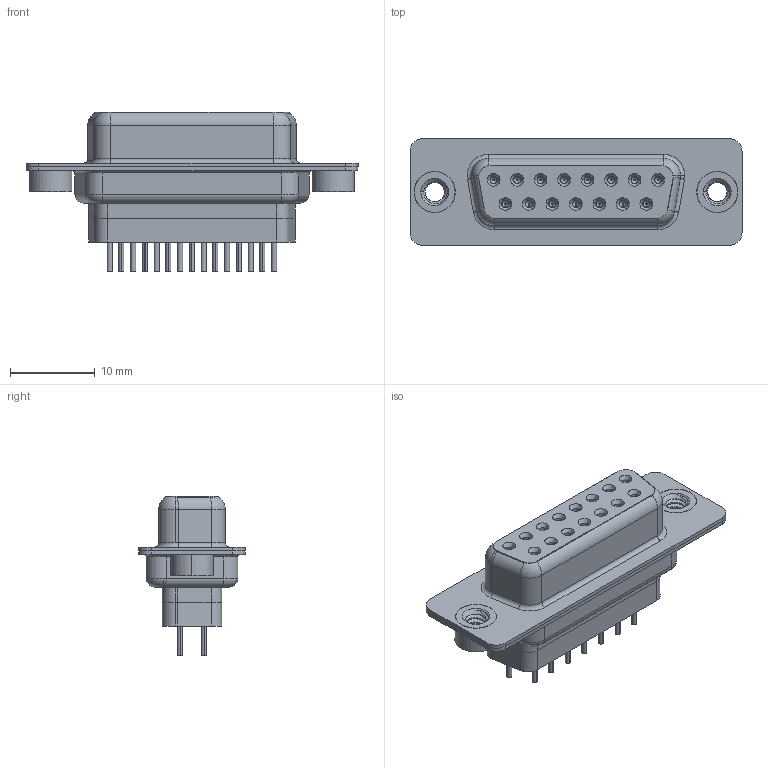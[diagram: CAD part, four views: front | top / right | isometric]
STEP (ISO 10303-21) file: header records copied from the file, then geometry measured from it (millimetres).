
FILE_DESCRIPTION (( 'STEP AP203' ), '1' );
FILE_NAME ('628-015-228-262.STEP', '2020-07-20T23:10:51', ( '' ), ( '' ), 'SwSTEP 2.0', 'SolidWorks 2020', '' );
FILE_SCHEMA (( 'CONFIG_CONTROL_DESIGN' ));
Length unit declared in the file: millimetre
Products named in the file (7): 628 Contact Row 1_28L; 628 Contact Row 2_28L; 628-015-228-262; 628 Shell Front_15 Contacts; 628 Housing_15 FF; 628 Shell Rear_15 Contacts; 628 4-40 Threaded Rivet
Assembly tree (20 placements, depth 2):
  628-015-228-262
    628 Housing_15 FF
    628 Shell Front_15 Contacts
    628 Shell Rear_15 Contacts
    628 Contact Row 1_28L  x8
    628 Contact Row 2_28L  x7
    628 4-40 Threaded Rivet  x2
Bounding box: 39.15 x 12.6 x 18.8 mm (x, y, z)
Volume: 2911.8 mm3; surface area: 7025.8 mm2
Topology: 21 solids, 21 shells, 2221 faces, 5652 edges, 3514 vertices
Faces by surface type: cylinder 665, plane 538, torus 447, bspline 306, cone 265
Entity records: 25385 total; most frequent: CARTESIAN_POINT 7532, DIRECTION 3643, ORIENTED_EDGE 3436, EDGE_CURVE 1718, AXIS2_PLACEMENT_3D 1514, VERTEX_POINT 1082, EDGE_LOOP 832, CIRCLE 830
